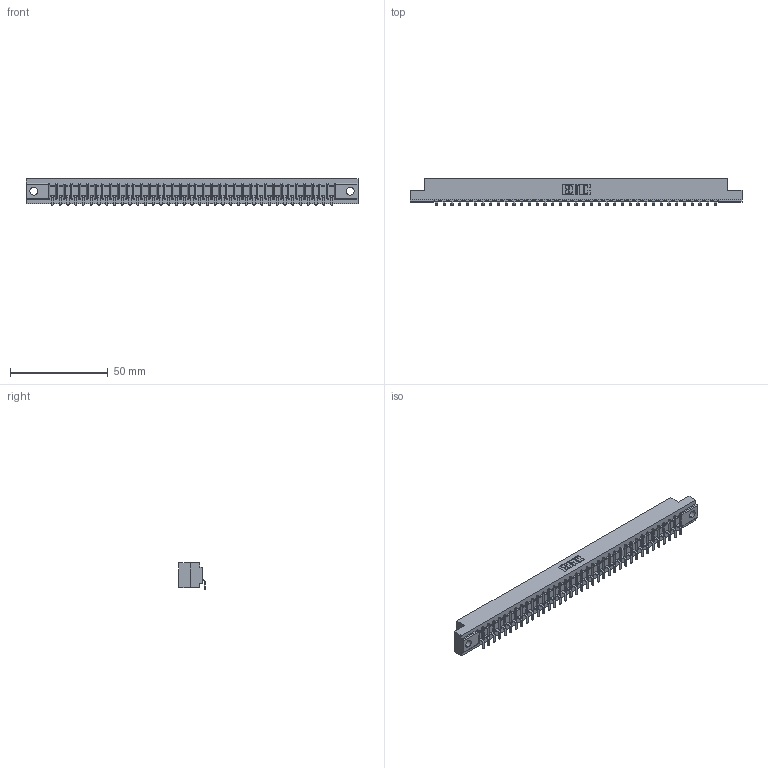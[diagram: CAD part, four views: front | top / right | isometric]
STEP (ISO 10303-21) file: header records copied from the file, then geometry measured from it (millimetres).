
FILE_DESCRIPTION (( 'STEP AP203' ), '1' );
FILE_NAME ('307-037-553-104.STEP', '2019-09-05T08:32:37', ( '' ), ( '' ), 'SwSTEP 2.0', 'SolidWorks 2016', '' );
FILE_SCHEMA (( 'CONFIG_CONTROL_DESIGN' ));
Length unit declared in the file: inch
Products named in the file (3): 307-290-002_553; 307 Part_.156 Dia Mounting Holes; 307-037-553-104
Assembly tree (38 placements, depth 2):
  307-037-553-104
    307 Part_.156 Dia Mounting Holes
    307-290-002_553  x37
Bounding box: 169.62 x 13.32 x 13.5 mm (x, y, z)
Volume: 18008.2 mm3; surface area: 22363 mm2
Topology: 38 solids, 38 shells, 3056 faces, 9387 edges, 6154 vertices
Faces by surface type: plane 1823, cylinder 1157, sphere 76
Entity records: 33608 total; most frequent: CARTESIAN_POINT 5674, ORIENTED_EDGE 5662, DIRECTION 5507, EDGE_CURVE 2831, VECTOR 2173, LINE 2173, VERTEX_POINT 1834, AXIS2_PLACEMENT_3D 1667
